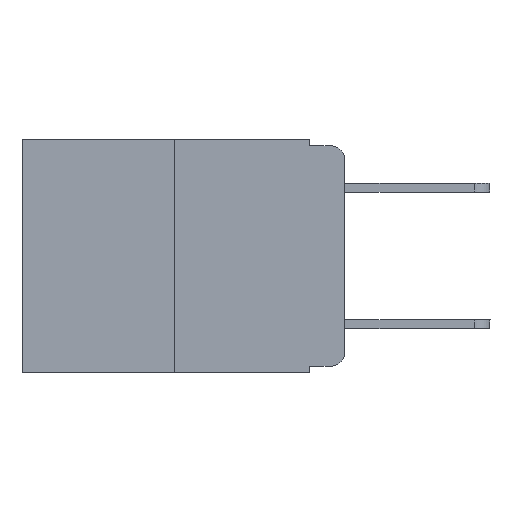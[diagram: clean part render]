
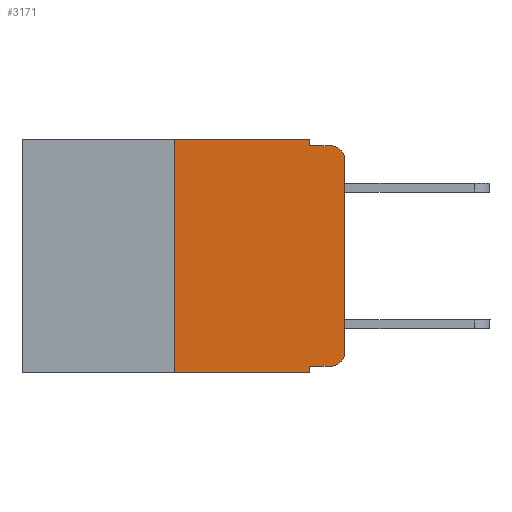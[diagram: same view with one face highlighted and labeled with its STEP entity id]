
A CAD part, left-side view. The second image highlights one B-rep face of the part: STEP entity #3171.
In plain terms, the highlighted planar face has unit normal (-1, 0, 0).
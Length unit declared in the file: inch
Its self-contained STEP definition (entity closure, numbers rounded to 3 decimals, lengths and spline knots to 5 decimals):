
#289 = CARTESIAN_POINT ( 'NONE',  ( 0., 0.02, -0.313 ) ) ;
#575 = CARTESIAN_POINT ( 'NONE',  ( 0., 0.25, 0. ) ) ;
#796 = VERTEX_POINT ( 'NONE', #1093 ) ;
#814 = LINE ( 'NONE', #7410, #7873 ) ;
#1001 = VERTEX_POINT ( 'NONE', #2075 ) ;
#1070 = EDGE_CURVE ( 'NONE', #10163, #796, #7084, .T. ) ;
#1073 = CARTESIAN_POINT ( 'NONE',  ( 0., 0.473, 0. ) ) ;
#1093 = CARTESIAN_POINT ( 'NONE',  ( 0., 0.051, -0.01 ) ) ;
#1321 = DIRECTION ( 'NONE',  ( 0., -1., 0. ) ) ;
#1332 = VERTEX_POINT ( 'NONE', #9651 ) ;
#1722 = LINE ( 'NONE', #1073, #11043 ) ;
#1839 = ORIENTED_EDGE ( 'NONE', *, *, #5180, .F. ) ;
#2075 = CARTESIAN_POINT ( 'NONE',  ( 0., 0.25, -0.343 ) ) ;
#2162 = EDGE_CURVE ( 'NONE', #1001, #5216, #7765, .T. ) ;
#2314 = ORIENTED_EDGE ( 'NONE', *, *, #9665, .T. ) ;
#2322 = VERTEX_POINT ( 'NONE', #9807 ) ;
#2605 = LINE ( 'NONE', #8330, #8802 ) ;
#2684 = VERTEX_POINT ( 'NONE', #6007 ) ;
#2699 = CARTESIAN_POINT ( 'NONE',  ( 0., 0.051, 0. ) ) ;
#2779 = PLANE ( 'NONE',  #5707 ) ;
#2817 = CARTESIAN_POINT ( 'NONE',  ( 0., 0.473, 0. ) ) ;
#2936 = EDGE_CURVE ( 'NONE', #1001, #1332, #4510, .T. ) ;
#2979 = CARTESIAN_POINT ( 'NONE',  ( 0., 0.051, -0.01 ) ) ;
#3171 = ADVANCED_FACE ( 'NONE', ( #8452 ), #2779, .F. ) ;
#3220 = EDGE_CURVE ( 'NONE', #4714, #2322, #4782, .T. ) ;
#3505 = DIRECTION ( 'NONE',  ( 0., -1., 0. ) ) ;
#3656 = VECTOR ( 'NONE', #3505, 39.37008 ) ;
#3703 = EDGE_CURVE ( 'NONE', #2322, #2684, #2605, .T. ) ;
#3872 = DIRECTION ( 'NONE',  ( 0., 0., -1. ) ) ;
#4005 = CARTESIAN_POINT ( 'NONE',  ( 0., 0.02, -0.03 ) ) ;
#4167 = DIRECTION ( 'NONE',  ( 0., 0., 1. ) ) ;
#4171 = ORIENTED_EDGE ( 'NONE', *, *, #2162, .F. ) ;
#4364 = VECTOR ( 'NONE', #8623, 39.37008 ) ;
#4510 = LINE ( 'NONE', #5835, #4364 ) ;
#4700 = VECTOR ( 'NONE', #3872, 39.37008 ) ;
#4714 = VERTEX_POINT ( 'NONE', #6035 ) ;
#4733 = EDGE_LOOP ( 'NONE', ( #5278, #2314, #1839, #7100, #9912, #4171, #10974, #6815, #11139, #8369 ) ) ;
#4782 = CIRCLE ( 'NONE', #6083, 0.02 ) ;
#5072 = LINE ( 'NONE', #10563, #3656 ) ;
#5180 = EDGE_CURVE ( 'NONE', #796, #9577, #11628, .T. ) ;
#5216 = VERTEX_POINT ( 'NONE', #8457 ) ;
#5278 = ORIENTED_EDGE ( 'NONE', *, *, #3703, .T. ) ;
#5386 = VECTOR ( 'NONE', #4167, 39.37008 ) ;
#5418 = VECTOR ( 'NONE', #1321, 39.37008 ) ;
#5707 = AXIS2_PLACEMENT_3D ( 'NONE', #2817, #9040, #10066 ) ;
#5712 = EDGE_CURVE ( 'NONE', #5216, #10163, #1722, .T. ) ;
#5835 = CARTESIAN_POINT ( 'NONE',  ( 0., 0.473, -0.343 ) ) ;
#6007 = CARTESIAN_POINT ( 'NONE',  ( 0., 0., -0.03 ) ) ;
#6035 = CARTESIAN_POINT ( 'NONE',  ( 0., 0.02, -0.333 ) ) ;
#6083 = AXIS2_PLACEMENT_3D ( 'NONE', #289, #9316, #11134 ) ;
#6194 = DIRECTION ( 'NONE',  ( -1., 0., 0. ) ) ;
#6601 = CARTESIAN_POINT ( 'NONE',  ( 0., 0.051, -0.333 ) ) ;
#6683 = CARTESIAN_POINT ( 'NONE',  ( 0., 0.02, -0.01 ) ) ;
#6815 = ORIENTED_EDGE ( 'NONE', *, *, #8388, .F. ) ;
#7084 = LINE ( 'NONE', #8360, #4700 ) ;
#7100 = ORIENTED_EDGE ( 'NONE', *, *, #1070, .F. ) ;
#7410 = CARTESIAN_POINT ( 'NONE',  ( 0., 0.051, 0. ) ) ;
#7411 = EDGE_CURVE ( 'NONE', #10458, #4714, #5072, .T. ) ;
#7519 = DIRECTION ( 'NONE',  ( 0., 0., -1. ) ) ;
#7765 = LINE ( 'NONE', #575, #5386 ) ;
#7873 = VECTOR ( 'NONE', #7519, 39.37008 ) ;
#8330 = CARTESIAN_POINT ( 'NONE',  ( 0., 0., 0. ) ) ;
#8360 = CARTESIAN_POINT ( 'NONE',  ( 0., 0.051, 0. ) ) ;
#8369 = ORIENTED_EDGE ( 'NONE', *, *, #3220, .T. ) ;
#8388 = EDGE_CURVE ( 'NONE', #10458, #1332, #814, .T. ) ;
#8452 = FACE_OUTER_BOUND ( 'NONE', #4733, .T. ) ;
#8457 = CARTESIAN_POINT ( 'NONE',  ( 0., 0.25, 0. ) ) ;
#8623 = DIRECTION ( 'NONE',  ( 0., -1., 0. ) ) ;
#8802 = VECTOR ( 'NONE', #9309, 39.37008 ) ;
#9003 = AXIS2_PLACEMENT_3D ( 'NONE', #4005, #6194, #10382 ) ;
#9040 = DIRECTION ( 'NONE',  ( 1., 0., 0. ) ) ;
#9309 = DIRECTION ( 'NONE',  ( 0., 0., 1. ) ) ;
#9316 = DIRECTION ( 'NONE',  ( -1., 0., 0. ) ) ;
#9577 = VERTEX_POINT ( 'NONE', #6683 ) ;
#9651 = CARTESIAN_POINT ( 'NONE',  ( 0., 0.051, -0.343 ) ) ;
#9665 = EDGE_CURVE ( 'NONE', #2684, #9577, #9813, .T. ) ;
#9807 = CARTESIAN_POINT ( 'NONE',  ( 0., 0., -0.313 ) ) ;
#9813 = CIRCLE ( 'NONE', #9003, 0.02 ) ;
#9912 = ORIENTED_EDGE ( 'NONE', *, *, #5712, .F. ) ;
#10066 = DIRECTION ( 'NONE',  ( 0., 0., -1. ) ) ;
#10163 = VERTEX_POINT ( 'NONE', #2699 ) ;
#10168 = DIRECTION ( 'NONE',  ( 0., -1., 0. ) ) ;
#10382 = DIRECTION ( 'NONE',  ( 0., 0., -1. ) ) ;
#10458 = VERTEX_POINT ( 'NONE', #6601 ) ;
#10563 = CARTESIAN_POINT ( 'NONE',  ( 0., 0.051, -0.333 ) ) ;
#10974 = ORIENTED_EDGE ( 'NONE', *, *, #2936, .T. ) ;
#11043 = VECTOR ( 'NONE', #10168, 39.37008 ) ;
#11134 = DIRECTION ( 'NONE',  ( 0., 0., -1. ) ) ;
#11139 = ORIENTED_EDGE ( 'NONE', *, *, #7411, .T. ) ;
#11628 = LINE ( 'NONE', #2979, #5418 ) ;
